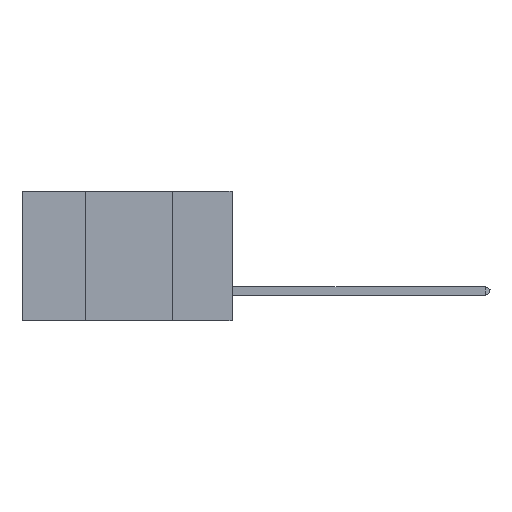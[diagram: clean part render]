
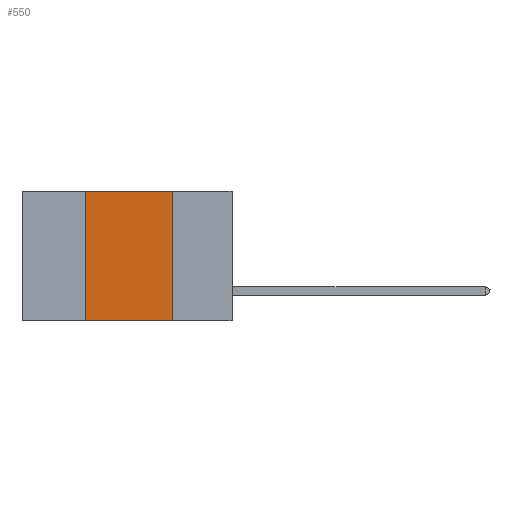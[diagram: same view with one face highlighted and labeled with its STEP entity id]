
A CAD part, left-side view. The second image highlights one B-rep face of the part: STEP entity #550.
In plain terms, the highlighted planar face has unit normal (-1, 0, 0).
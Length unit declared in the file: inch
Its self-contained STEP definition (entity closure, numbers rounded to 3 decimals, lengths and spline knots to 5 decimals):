
#550 = ADVANCED_FACE ( 'NONE', ( #4162 ), #12001, .F. ) ;
#582 = ORIENTED_EDGE ( 'NONE', *, *, #5883, .F. ) ;
#1388 = CARTESIAN_POINT ( 'NONE',  ( 0., 0.42, 0. ) ) ;
#1624 = VECTOR ( 'NONE', #7565, 39.37008 ) ;
#2084 = DIRECTION ( 'NONE',  ( 1., 0., 0. ) ) ;
#2382 = LINE ( 'NONE', #14073, #11549 ) ;
#2696 = CARTESIAN_POINT ( 'NONE',  ( 0., 0.17, -0.37 ) ) ;
#4162 = FACE_OUTER_BOUND ( 'NONE', #12657, .T. ) ;
#4207 = CARTESIAN_POINT ( 'NONE',  ( 0., 0.42, -0.37 ) ) ;
#5270 = LINE ( 'NONE', #7426, #1624 ) ;
#5276 = CARTESIAN_POINT ( 'NONE',  ( 0., 0.6, 0. ) ) ;
#5778 = EDGE_CURVE ( 'NONE', #11507, #7405, #8780, .T. ) ;
#5883 = EDGE_CURVE ( 'NONE', #9538, #13427, #2382, .T. ) ;
#5994 = AXIS2_PLACEMENT_3D ( 'NONE', #5276, #2084, #13084 ) ;
#6004 = ORIENTED_EDGE ( 'NONE', *, *, #5778, .T. ) ;
#6475 = EDGE_CURVE ( 'NONE', #11507, #9538, #11150, .T. ) ;
#7126 = ORIENTED_EDGE ( 'NONE', *, *, #6475, .F. ) ;
#7405 = VERTEX_POINT ( 'NONE', #2696 ) ;
#7426 = CARTESIAN_POINT ( 'NONE',  ( 0., 0.17, 0. ) ) ;
#7461 = DIRECTION ( 'NONE',  ( 0., -1., 0. ) ) ;
#7565 = DIRECTION ( 'NONE',  ( 0., 0., -1. ) ) ;
#8180 = CARTESIAN_POINT ( 'NONE',  ( 0., 0.6, -0.37 ) ) ;
#8780 = LINE ( 'NONE', #8180, #9834 ) ;
#9538 = VERTEX_POINT ( 'NONE', #1388 ) ;
#9622 = VECTOR ( 'NONE', #10340, 39.37008 ) ;
#9651 = CARTESIAN_POINT ( 'NONE',  ( 0., 0.17, 0. ) ) ;
#9834 = VECTOR ( 'NONE', #10445, 39.37008 ) ;
#10340 = DIRECTION ( 'NONE',  ( 0., 0., 1. ) ) ;
#10445 = DIRECTION ( 'NONE',  ( 0., -1., 0. ) ) ;
#11150 = LINE ( 'NONE', #11461, #9622 ) ;
#11461 = CARTESIAN_POINT ( 'NONE',  ( 0., 0.42, 0. ) ) ;
#11507 = VERTEX_POINT ( 'NONE', #4207 ) ;
#11549 = VECTOR ( 'NONE', #7461, 39.37008 ) ;
#11704 = ORIENTED_EDGE ( 'NONE', *, *, #13323, .F. ) ;
#12001 = PLANE ( 'NONE',  #5994 ) ;
#12657 = EDGE_LOOP ( 'NONE', ( #11704, #582, #7126, #6004 ) ) ;
#13084 = DIRECTION ( 'NONE',  ( 0., 0., -1. ) ) ;
#13323 = EDGE_CURVE ( 'NONE', #13427, #7405, #5270, .T. ) ;
#13427 = VERTEX_POINT ( 'NONE', #9651 ) ;
#14073 = CARTESIAN_POINT ( 'NONE',  ( 0., 0.6, 0. ) ) ;
